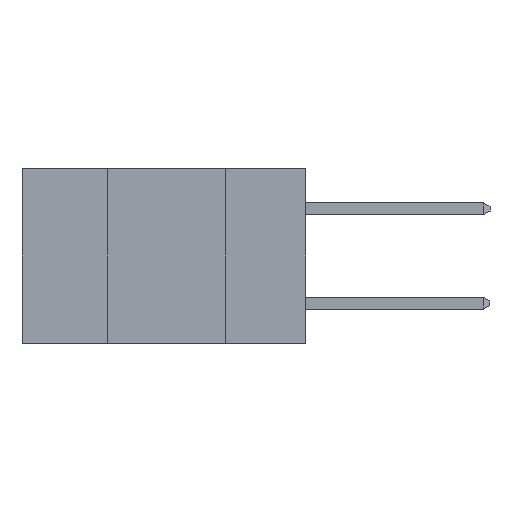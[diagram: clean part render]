
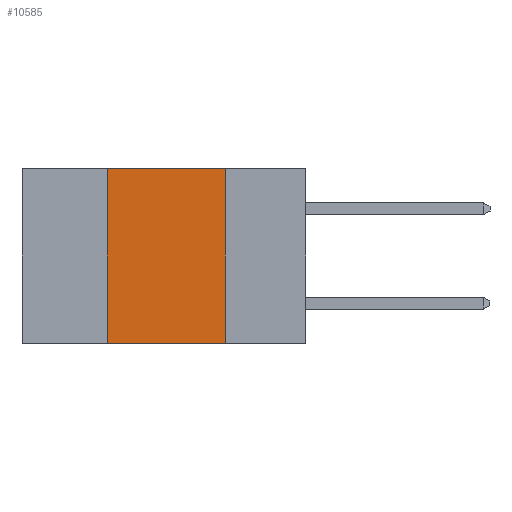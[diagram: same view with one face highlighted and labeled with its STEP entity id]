
A CAD part, left-side view. The second image highlights one B-rep face of the part: STEP entity #10585.
In plain terms, the highlighted planar face has unit normal (-1, 0, 0).
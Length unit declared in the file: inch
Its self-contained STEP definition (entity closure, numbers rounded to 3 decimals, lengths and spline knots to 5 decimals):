
#93 = LINE ( 'NONE', #24633, #14925 ) ;
#960 = CARTESIAN_POINT ( 'NONE',  ( 0., 0.42, -0.37 ) ) ;
#2776 = VECTOR ( 'NONE', #3801, 39.37008 ) ;
#2818 = EDGE_CURVE ( 'NONE', #8930, #16309, #93, .T. ) ;
#3801 = DIRECTION ( 'NONE',  ( 0., 0., 1. ) ) ;
#4485 = VERTEX_POINT ( 'NONE', #4820 ) ;
#4820 = CARTESIAN_POINT ( 'NONE',  ( 0., 0.17, -0.37 ) ) ;
#6020 = EDGE_CURVE ( 'NONE', #9054, #4485, #15648, .T. ) ;
#6031 = EDGE_LOOP ( 'NONE', ( #18864, #18602, #6890, #15164 ) ) ;
#6491 = CARTESIAN_POINT ( 'NONE',  ( 0., 0.42, 0. ) ) ;
#6890 = ORIENTED_EDGE ( 'NONE', *, *, #10335, .F. ) ;
#8217 = CARTESIAN_POINT ( 'NONE',  ( 0., 0.17, 0. ) ) ;
#8404 = DIRECTION ( 'NONE',  ( 1., 0., 0. ) ) ;
#8930 = VERTEX_POINT ( 'NONE', #6491 ) ;
#9054 = VERTEX_POINT ( 'NONE', #960 ) ;
#9519 = AXIS2_PLACEMENT_3D ( 'NONE', #14127, #8404, #21770 ) ;
#10335 = EDGE_CURVE ( 'NONE', #9054, #8930, #16387, .T. ) ;
#10585 = ADVANCED_FACE ( 'NONE', ( #19940 ), #17954, .F. ) ;
#13119 = EDGE_CURVE ( 'NONE', #16309, #4485, #13318, .T. ) ;
#13318 = LINE ( 'NONE', #8217, #18369 ) ;
#14127 = CARTESIAN_POINT ( 'NONE',  ( 0., 0.6, 0. ) ) ;
#14925 = VECTOR ( 'NONE', #16254, 39.37008 ) ;
#15139 = CARTESIAN_POINT ( 'NONE',  ( 0., 0.6, -0.37 ) ) ;
#15164 = ORIENTED_EDGE ( 'NONE', *, *, #6020, .T. ) ;
#15648 = LINE ( 'NONE', #15139, #20700 ) ;
#16254 = DIRECTION ( 'NONE',  ( 0., -1., 0. ) ) ;
#16309 = VERTEX_POINT ( 'NONE', #19448 ) ;
#16387 = LINE ( 'NONE', #19218, #2776 ) ;
#17041 = DIRECTION ( 'NONE',  ( 0., -1., 0. ) ) ;
#17954 = PLANE ( 'NONE',  #9519 ) ;
#18369 = VECTOR ( 'NONE', #21586, 39.37008 ) ;
#18602 = ORIENTED_EDGE ( 'NONE', *, *, #2818, .F. ) ;
#18864 = ORIENTED_EDGE ( 'NONE', *, *, #13119, .F. ) ;
#19218 = CARTESIAN_POINT ( 'NONE',  ( 0., 0.42, 0. ) ) ;
#19448 = CARTESIAN_POINT ( 'NONE',  ( 0., 0.17, 0. ) ) ;
#19940 = FACE_OUTER_BOUND ( 'NONE', #6031, .T. ) ;
#20700 = VECTOR ( 'NONE', #17041, 39.37008 ) ;
#21586 = DIRECTION ( 'NONE',  ( 0., 0., -1. ) ) ;
#21770 = DIRECTION ( 'NONE',  ( 0., 0., -1. ) ) ;
#24633 = CARTESIAN_POINT ( 'NONE',  ( 0., 0.6, 0. ) ) ;
